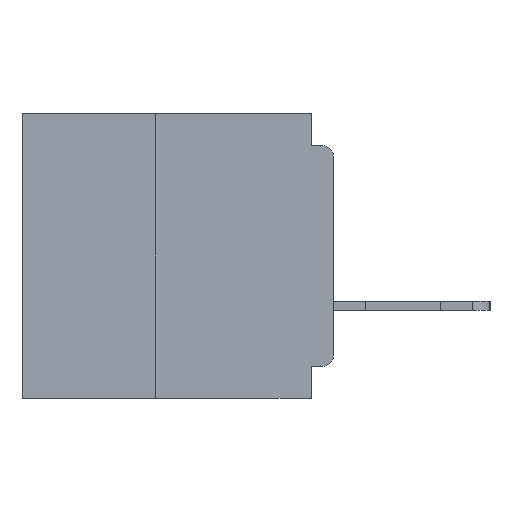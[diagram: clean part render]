
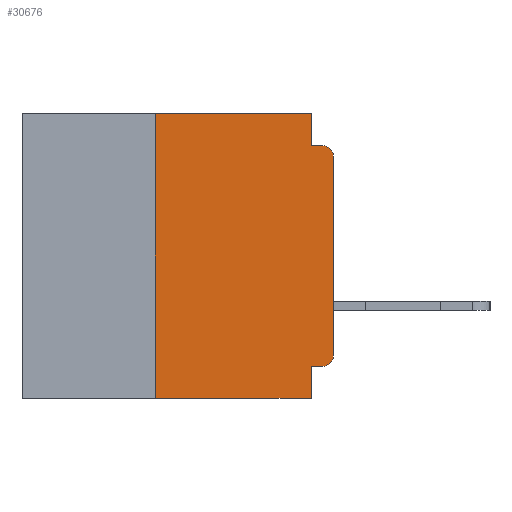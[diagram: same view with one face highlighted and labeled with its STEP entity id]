
A CAD part, left-side view. The second image highlights one B-rep face of the part: STEP entity #30676.
In plain terms, the highlighted planar face has unit normal (-1, 0, 0).
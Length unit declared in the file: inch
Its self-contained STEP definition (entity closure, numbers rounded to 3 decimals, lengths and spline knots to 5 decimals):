
#38 = VECTOR ( 'NONE', #21037, 39.37008 ) ;
#157 = VERTEX_POINT ( 'NONE', #36618 ) ;
#424 = CARTESIAN_POINT ( 'NONE',  ( 0., 0., 0. ) ) ;
#447 = CARTESIAN_POINT ( 'NONE',  ( 0., 0., -0.355 ) ) ;
#2156 = DIRECTION ( 'NONE',  ( 1., 0., 0. ) ) ;
#2499 = VECTOR ( 'NONE', #24002, 39.37008 ) ;
#2629 = EDGE_CURVE ( 'NONE', #3432, #16624, #5733, .T. ) ;
#2848 = ORIENTED_EDGE ( 'NONE', *, *, #21145, .T. ) ;
#3432 = VERTEX_POINT ( 'NONE', #21918 ) ;
#3805 = LINE ( 'NONE', #37275, #18602 ) ;
#4107 = DIRECTION ( 'NONE',  ( -1., 0., 0. ) ) ;
#5093 = CIRCLE ( 'NONE', #15974, 0.015 ) ;
#5318 = DIRECTION ( 'NONE',  ( -1., 0., 0. ) ) ;
#5733 = LINE ( 'NONE', #8491, #13608 ) ;
#5967 = DIRECTION ( 'NONE',  ( 0., -1., 0. ) ) ;
#6060 = VERTEX_POINT ( 'NONE', #16878 ) ;
#7026 = ORIENTED_EDGE ( 'NONE', *, *, #20414, .T. ) ;
#7131 = ORIENTED_EDGE ( 'NONE', *, *, #15278, .T. ) ;
#8491 = CARTESIAN_POINT ( 'NONE',  ( 0., 0., -0.045 ) ) ;
#8704 = CARTESIAN_POINT ( 'NONE',  ( 0., 0., -0.34 ) ) ;
#8746 = DIRECTION ( 'NONE',  ( 0., -1., 0. ) ) ;
#9571 = EDGE_CURVE ( 'NONE', #34996, #27563, #21096, .T. ) ;
#10303 = AXIS2_PLACEMENT_3D ( 'NONE', #19838, #2156, #22760 ) ;
#11569 = EDGE_CURVE ( 'NONE', #6060, #27563, #24583, .T. ) ;
#13608 = VECTOR ( 'NONE', #8746, 39.37008 ) ;
#13949 = PLANE ( 'NONE',  #10303 ) ;
#15278 = EDGE_CURVE ( 'NONE', #157, #19771, #5093, .T. ) ;
#15410 = ORIENTED_EDGE ( 'NONE', *, *, #15505, .F. ) ;
#15463 = DIRECTION ( 'NONE',  ( 0., 0., -1. ) ) ;
#15505 = EDGE_CURVE ( 'NONE', #6060, #21640, #26225, .T. ) ;
#15757 = CARTESIAN_POINT ( 'NONE',  ( 0., 0., -0.06 ) ) ;
#15974 = AXIS2_PLACEMENT_3D ( 'NONE', #22920, #5318, #25891 ) ;
#16360 = AXIS2_PLACEMENT_3D ( 'NONE', #21746, #4107, #24689 ) ;
#16624 = VERTEX_POINT ( 'NONE', #29369 ) ;
#16816 = VECTOR ( 'NONE', #5967, 39.37008 ) ;
#16878 = CARTESIAN_POINT ( 'NONE',  ( 0., 0.25, -0.4 ) ) ;
#17472 = EDGE_CURVE ( 'NONE', #30799, #3432, #18749, .T. ) ;
#18602 = VECTOR ( 'NONE', #37401, 39.37008 ) ;
#18749 = LINE ( 'NONE', #24135, #34203 ) ;
#18795 = VERTEX_POINT ( 'NONE', #15757 ) ;
#19052 = ORIENTED_EDGE ( 'NONE', *, *, #17472, .F. ) ;
#19293 = VECTOR ( 'NONE', #37188, 39.37008 ) ;
#19372 = CIRCLE ( 'NONE', #16360, 0.015 ) ;
#19375 = VECTOR ( 'NONE', #35617, 39.37008 ) ;
#19771 = VERTEX_POINT ( 'NONE', #8704 ) ;
#19838 = CARTESIAN_POINT ( 'NONE',  ( 0., 0.437, 0. ) ) ;
#20414 = EDGE_CURVE ( 'NONE', #19771, #18795, #29497, .T. ) ;
#21037 = DIRECTION ( 'NONE',  ( 0., 0., 1. ) ) ;
#21096 = LINE ( 'NONE', #25635, #19293 ) ;
#21145 = EDGE_CURVE ( 'NONE', #18795, #16624, #19372, .T. ) ;
#21594 = CARTESIAN_POINT ( 'NONE',  ( 0., 0.25, 0. ) ) ;
#21640 = VERTEX_POINT ( 'NONE', #21594 ) ;
#21746 = CARTESIAN_POINT ( 'NONE',  ( 0., 0.015, -0.06 ) ) ;
#21849 = ORIENTED_EDGE ( 'NONE', *, *, #27042, .F. ) ;
#21918 = CARTESIAN_POINT ( 'NONE',  ( 0., 0.031, -0.045 ) ) ;
#22760 = DIRECTION ( 'NONE',  ( 0., 0., -1. ) ) ;
#22920 = CARTESIAN_POINT ( 'NONE',  ( 0., 0.015, -0.34 ) ) ;
#23866 = FACE_OUTER_BOUND ( 'NONE', #34606, .T. ) ;
#24002 = DIRECTION ( 'NONE',  ( 0., 1., 0. ) ) ;
#24079 = CARTESIAN_POINT ( 'NONE',  ( 0., 0.031, -0.355 ) ) ;
#24135 = CARTESIAN_POINT ( 'NONE',  ( 0., 0.031, 0. ) ) ;
#24583 = LINE ( 'NONE', #29475, #16816 ) ;
#24689 = DIRECTION ( 'NONE',  ( 0., 0., -1. ) ) ;
#25635 = CARTESIAN_POINT ( 'NONE',  ( 0., 0.031, -0.4 ) ) ;
#25891 = DIRECTION ( 'NONE',  ( 0., 0., -1. ) ) ;
#26003 = LINE ( 'NONE', #447, #2499 ) ;
#26225 = LINE ( 'NONE', #32693, #19375 ) ;
#26405 = ORIENTED_EDGE ( 'NONE', *, *, #9571, .F. ) ;
#27042 = EDGE_CURVE ( 'NONE', #157, #34996, #26003, .T. ) ;
#27563 = VERTEX_POINT ( 'NONE', #32223 ) ;
#28062 = EDGE_CURVE ( 'NONE', #21640, #30799, #3805, .T. ) ;
#28233 = ORIENTED_EDGE ( 'NONE', *, *, #28062, .F. ) ;
#29369 = CARTESIAN_POINT ( 'NONE',  ( 0., 0.015, -0.045 ) ) ;
#29475 = CARTESIAN_POINT ( 'NONE',  ( 0., 0.437, -0.4 ) ) ;
#29497 = LINE ( 'NONE', #424, #38 ) ;
#29612 = ORIENTED_EDGE ( 'NONE', *, *, #11569, .T. ) ;
#30676 = ADVANCED_FACE ( 'NONE', ( #23866 ), #13949, .F. ) ;
#30799 = VERTEX_POINT ( 'NONE', #37766 ) ;
#32223 = CARTESIAN_POINT ( 'NONE',  ( 0., 0.031, -0.4 ) ) ;
#32693 = CARTESIAN_POINT ( 'NONE',  ( 0., 0.25, -0.4 ) ) ;
#34203 = VECTOR ( 'NONE', #15463, 39.37008 ) ;
#34606 = EDGE_LOOP ( 'NONE', ( #7026, #2848, #35855, #19052, #28233, #15410, #29612, #26405, #21849, #7131 ) ) ;
#34996 = VERTEX_POINT ( 'NONE', #24079 ) ;
#35617 = DIRECTION ( 'NONE',  ( 0., 0., 1. ) ) ;
#35855 = ORIENTED_EDGE ( 'NONE', *, *, #2629, .F. ) ;
#36618 = CARTESIAN_POINT ( 'NONE',  ( 0., 0.015, -0.355 ) ) ;
#37188 = DIRECTION ( 'NONE',  ( 0., 0., -1. ) ) ;
#37275 = CARTESIAN_POINT ( 'NONE',  ( 0., 0.437, 0. ) ) ;
#37401 = DIRECTION ( 'NONE',  ( 0., -1., 0. ) ) ;
#37766 = CARTESIAN_POINT ( 'NONE',  ( 0., 0.031, 0. ) ) ;
